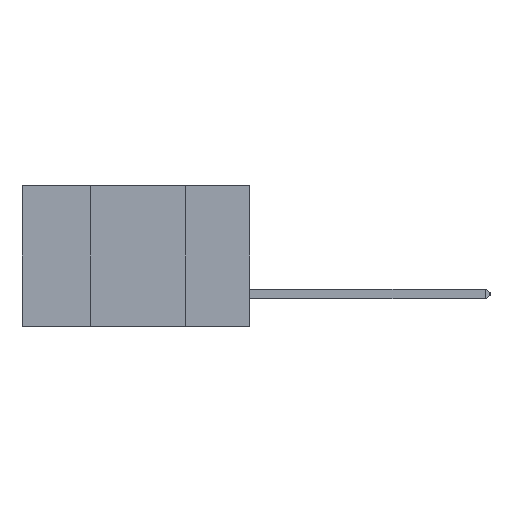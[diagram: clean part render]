
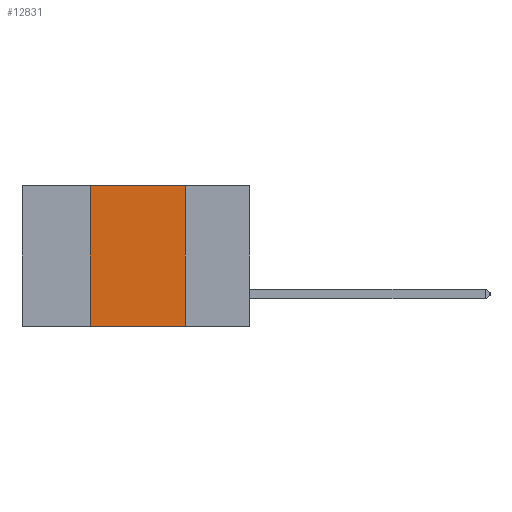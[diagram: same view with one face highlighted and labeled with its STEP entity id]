
A CAD part, left-side view. The second image highlights one B-rep face of the part: STEP entity #12831.
In plain terms, the highlighted planar face has unit normal (-1, 0, 0).
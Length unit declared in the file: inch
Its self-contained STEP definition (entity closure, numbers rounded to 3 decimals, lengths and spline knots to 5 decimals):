
#600 = LINE ( 'NONE', #17428, #11060 ) ;
#867 = LINE ( 'NONE', #1453, #17255 ) ;
#1453 = CARTESIAN_POINT ( 'NONE',  ( 0., 0.42, 0. ) ) ;
#1553 = EDGE_CURVE ( 'NONE', #15849, #17602, #867, .T. ) ;
#3781 = ORIENTED_EDGE ( 'NONE', *, *, #17222, .T. ) ;
#4999 = CARTESIAN_POINT ( 'NONE',  ( 0., 0.6, -0.37 ) ) ;
#8058 = ORIENTED_EDGE ( 'NONE', *, *, #12369, .F. ) ;
#9627 = PLANE ( 'NONE',  #14582 ) ;
#10041 = CARTESIAN_POINT ( 'NONE',  ( 0., 0.17, -0.37 ) ) ;
#10210 = ORIENTED_EDGE ( 'NONE', *, *, #16730, .F. ) ;
#11060 = VECTOR ( 'NONE', #19048, 39.37008 ) ;
#12269 = VECTOR ( 'NONE', #16585, 39.37008 ) ;
#12369 = EDGE_CURVE ( 'NONE', #17602, #15580, #17019, .T. ) ;
#12811 = DIRECTION ( 'NONE',  ( 1., 0., 0. ) ) ;
#12831 = ADVANCED_FACE ( 'NONE', ( #17520 ), #9627, .F. ) ;
#12958 = DIRECTION ( 'NONE',  ( 0., 0., -1. ) ) ;
#13580 = VECTOR ( 'NONE', #15563, 39.37008 ) ;
#14288 = DIRECTION ( 'NONE',  ( 0., 0., 1. ) ) ;
#14582 = AXIS2_PLACEMENT_3D ( 'NONE', #17623, #12811, #12958 ) ;
#15563 = DIRECTION ( 'NONE',  ( 0., -1., 0. ) ) ;
#15580 = VERTEX_POINT ( 'NONE', #18975 ) ;
#15849 = VERTEX_POINT ( 'NONE', #18448 ) ;
#16585 = DIRECTION ( 'NONE',  ( 0., -1., 0. ) ) ;
#16730 = EDGE_CURVE ( 'NONE', #15580, #20048, #600, .T. ) ;
#16850 = CARTESIAN_POINT ( 'NONE',  ( 0., 0.42, 0. ) ) ;
#17002 = CARTESIAN_POINT ( 'NONE',  ( 0., 0.6, 0. ) ) ;
#17019 = LINE ( 'NONE', #17002, #13580 ) ;
#17222 = EDGE_CURVE ( 'NONE', #15849, #20048, #18772, .T. ) ;
#17255 = VECTOR ( 'NONE', #14288, 39.37008 ) ;
#17428 = CARTESIAN_POINT ( 'NONE',  ( 0., 0.17, 0. ) ) ;
#17520 = FACE_OUTER_BOUND ( 'NONE', #19274, .T. ) ;
#17602 = VERTEX_POINT ( 'NONE', #16850 ) ;
#17623 = CARTESIAN_POINT ( 'NONE',  ( 0., 0.6, 0. ) ) ;
#18448 = CARTESIAN_POINT ( 'NONE',  ( 0., 0.42, -0.37 ) ) ;
#18772 = LINE ( 'NONE', #4999, #12269 ) ;
#18975 = CARTESIAN_POINT ( 'NONE',  ( 0., 0.17, 0. ) ) ;
#19048 = DIRECTION ( 'NONE',  ( 0., 0., -1. ) ) ;
#19274 = EDGE_LOOP ( 'NONE', ( #10210, #8058, #19889, #3781 ) ) ;
#19889 = ORIENTED_EDGE ( 'NONE', *, *, #1553, .F. ) ;
#20048 = VERTEX_POINT ( 'NONE', #10041 ) ;
